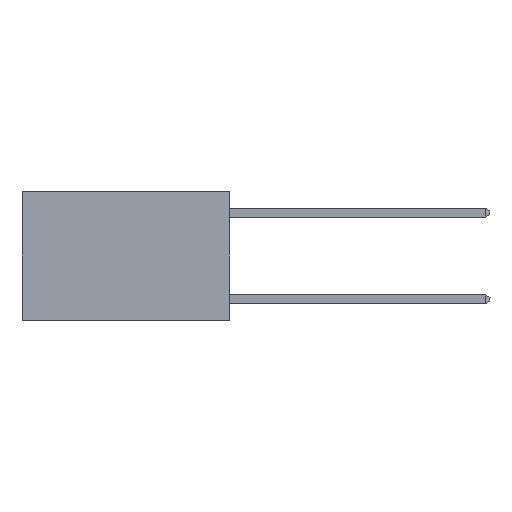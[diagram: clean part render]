
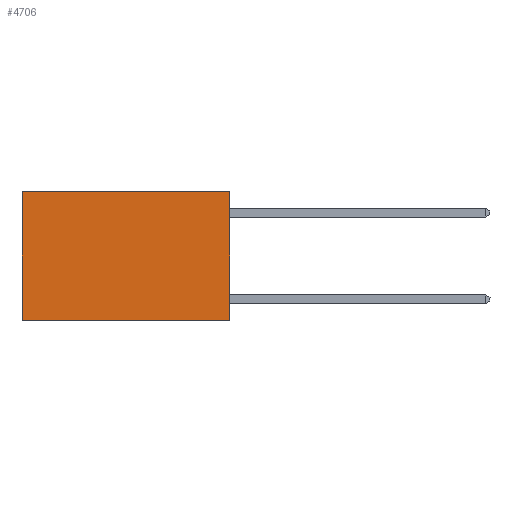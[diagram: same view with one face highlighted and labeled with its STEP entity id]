
A CAD part, left-side view. The second image highlights one B-rep face of the part: STEP entity #4706.
In plain terms, the highlighted planar face has unit normal (-1, 0, 0).
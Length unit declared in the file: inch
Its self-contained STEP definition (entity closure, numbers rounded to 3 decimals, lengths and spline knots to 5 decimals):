
#138 = VERTEX_POINT ( 'NONE', #4981 ) ;
#171 = DIRECTION ( 'NONE',  ( 1., 0., 0. ) ) ;
#346 = AXIS2_PLACEMENT_3D ( 'NONE', #2328, #171, #5058 ) ;
#439 = ORIENTED_EDGE ( 'NONE', *, *, #4423, .T. ) ;
#463 = LINE ( 'NONE', #7832, #5710 ) ;
#476 = CARTESIAN_POINT ( 'NONE',  ( 0.2625, 0.6, 0. ) ) ;
#645 = VECTOR ( 'NONE', #1222, 39.37008 ) ;
#1222 = DIRECTION ( 'NONE',  ( 0., 0., -1. ) ) ;
#1251 = DIRECTION ( 'NONE',  ( 0., 1., 0. ) ) ;
#1320 = VERTEX_POINT ( 'NONE', #7140 ) ;
#1776 = FACE_OUTER_BOUND ( 'NONE', #5718, .T. ) ;
#1817 = ORIENTED_EDGE ( 'NONE', *, *, #4384, .T. ) ;
#2118 = VECTOR ( 'NONE', #1251, 39.37008 ) ;
#2328 = CARTESIAN_POINT ( 'NONE',  ( 0.2625, 0., 0. ) ) ;
#2555 = LINE ( 'NONE', #5962, #2118 ) ;
#2871 = ORIENTED_EDGE ( 'NONE', *, *, #5318, .F. ) ;
#3174 = DIRECTION ( 'NONE',  ( 0., 0., -1. ) ) ;
#3456 = LINE ( 'NONE', #7663, #6719 ) ;
#4000 = CARTESIAN_POINT ( 'NONE',  ( 0.2625, 0., 0. ) ) ;
#4355 = LINE ( 'NONE', #476, #645 ) ;
#4379 = DIRECTION ( 'NONE',  ( 0., 1., 0. ) ) ;
#4384 = EDGE_CURVE ( 'NONE', #1320, #138, #4355, .T. ) ;
#4423 = EDGE_CURVE ( 'NONE', #8076, #1320, #2555, .T. ) ;
#4481 = ORIENTED_EDGE ( 'NONE', *, *, #5482, .F. ) ;
#4706 = ADVANCED_FACE ( 'NONE', ( #1776 ), #6943, .F. ) ;
#4981 = CARTESIAN_POINT ( 'NONE',  ( 0.2625, 0.6, -0.37 ) ) ;
#5058 = DIRECTION ( 'NONE',  ( 0., 0., -1. ) ) ;
#5318 = EDGE_CURVE ( 'NONE', #5631, #138, #3456, .T. ) ;
#5482 = EDGE_CURVE ( 'NONE', #8076, #5631, #463, .T. ) ;
#5631 = VERTEX_POINT ( 'NONE', #6548 ) ;
#5710 = VECTOR ( 'NONE', #3174, 39.37008 ) ;
#5718 = EDGE_LOOP ( 'NONE', ( #1817, #2871, #4481, #439 ) ) ;
#5962 = CARTESIAN_POINT ( 'NONE',  ( 0.2625, 0., 0. ) ) ;
#6548 = CARTESIAN_POINT ( 'NONE',  ( 0.2625, 0., -0.37 ) ) ;
#6719 = VECTOR ( 'NONE', #4379, 39.37008 ) ;
#6943 = PLANE ( 'NONE',  #346 ) ;
#7140 = CARTESIAN_POINT ( 'NONE',  ( 0.2625, 0.6, 0. ) ) ;
#7663 = CARTESIAN_POINT ( 'NONE',  ( 0.2625, 0., -0.37 ) ) ;
#7832 = CARTESIAN_POINT ( 'NONE',  ( 0.2625, 0., 0. ) ) ;
#8076 = VERTEX_POINT ( 'NONE', #4000 ) ;
